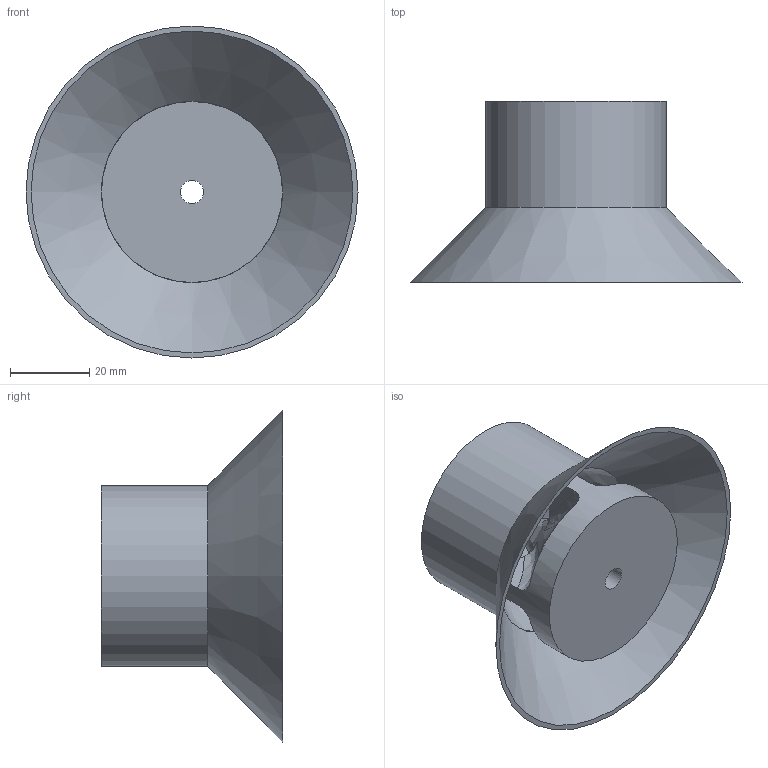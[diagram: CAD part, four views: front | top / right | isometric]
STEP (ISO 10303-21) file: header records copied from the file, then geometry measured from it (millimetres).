
FILE_DESCRIPTION(/* description */ (''),/* implementation_level */ '2;1');
FILE_NAME(/* name */ '1.8 Dia 23 CAL Baffle STEP.step',/* time_stamp */ '2019-06-09T15:37:06-04:00',/* author */ (''),/* organization */ (''),/* preprocessor_version */ 'ST-DEVELOPER v18',/* originating_system */ 'Autodesk Translation Framework v8.2.0.1029',/* authorisation */ '');
FILE_SCHEMA (('AUTOMOTIVE_DESIGN { 1 0 10303 214 3 1 1 }'));
Length unit declared in the file: inch
Products named in the file (1): baf 7
Bounding box: 83.82 x 45.72 x 83.82 mm (x, y, z)
Volume: 58079.6 mm3; surface area: 25238.2 mm2
Topology: 1 solids, 1 shells, 40 faces, 145 edges, 100 vertices
Faces by surface type: plane 15, bspline 14, cylinder 8, cone 2, torus 1
Full cylindrical faces by diameter (mm): 5.842 x2, 45.72 x2
Entity records: 2784 total; most frequent: CARTESIAN_POINT 1665, ORIENTED_EDGE 290, DIRECTION 154, EDGE_CURVE 145, VERTEX_POINT 100, B_SPLINE_CURVE_WITH_KNOTS 70, AXIS2_PLACEMENT_3D 62, EDGE_LOOP 43
